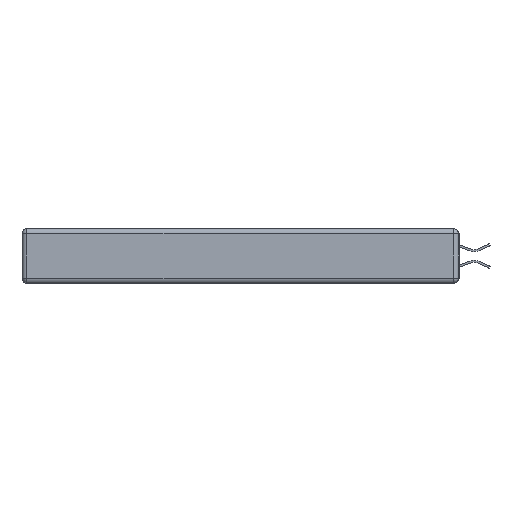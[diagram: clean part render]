
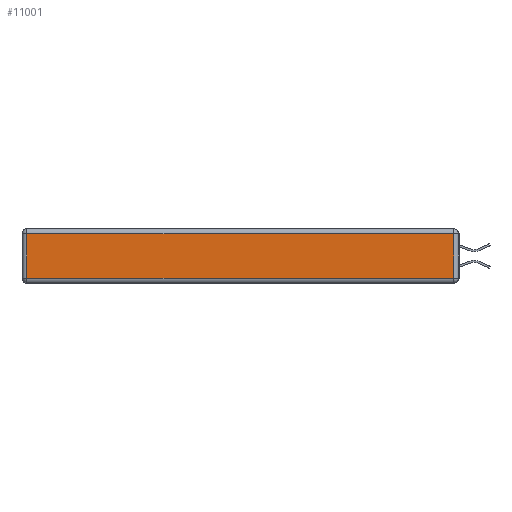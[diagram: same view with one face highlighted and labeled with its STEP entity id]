
A CAD part, left-side view. The second image highlights one B-rep face of the part: STEP entity #11001.
In plain terms, the highlighted planar face has unit normal (-1, 0, 0).
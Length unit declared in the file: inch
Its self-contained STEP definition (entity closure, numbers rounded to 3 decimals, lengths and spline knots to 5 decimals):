
#129 = LINE ( 'NONE', #2565, #17460 ) ;
#185 = FACE_OUTER_BOUND ( 'NONE', #7749, .T. ) ;
#680 = ORIENTED_EDGE ( 'NONE', *, *, #11595, .T. ) ;
#705 = VECTOR ( 'NONE', #15990, 39.37008 ) ;
#1683 = DIRECTION ( 'NONE',  ( 0., 0., -1. ) ) ;
#2207 = VECTOR ( 'NONE', #8833, 39.37008 ) ;
#2259 = CARTESIAN_POINT ( 'NONE',  ( 0., 0.03, -0.03 ) ) ;
#2486 = CARTESIAN_POINT ( 'NONE',  ( 0., 0.03, -0.343 ) ) ;
#2565 = CARTESIAN_POINT ( 'NONE',  ( 0., 2.72, -0.343 ) ) ;
#2656 = DIRECTION ( 'NONE',  ( -1., 0., 0. ) ) ;
#5015 = CARTESIAN_POINT ( 'NONE',  ( 0., 2.72, -0.03 ) ) ;
#5142 = ORIENTED_EDGE ( 'NONE', *, *, #6694, .T. ) ;
#6274 = EDGE_CURVE ( 'NONE', #8579, #17304, #129, .T. ) ;
#6694 = EDGE_CURVE ( 'NONE', #13769, #8579, #16343, .T. ) ;
#7749 = EDGE_LOOP ( 'NONE', ( #680, #15791, #5142, #9722 ) ) ;
#8579 = VERTEX_POINT ( 'NONE', #5015 ) ;
#8601 = LINE ( 'NONE', #2486, #705 ) ;
#8833 = DIRECTION ( 'NONE',  ( 0., 1., 0. ) ) ;
#9507 = AXIS2_PLACEMENT_3D ( 'NONE', #16330, #2656, #13450 ) ;
#9722 = ORIENTED_EDGE ( 'NONE', *, *, #6274, .T. ) ;
#9966 = VECTOR ( 'NONE', #14427, 39.37008 ) ;
#10369 = CARTESIAN_POINT ( 'NONE',  ( 0., 2.75, -0.03 ) ) ;
#11001 = ADVANCED_FACE ( 'NONE', ( #185 ), #17706, .T. ) ;
#11276 = VERTEX_POINT ( 'NONE', #16136 ) ;
#11595 = EDGE_CURVE ( 'NONE', #17304, #11276, #17279, .T. ) ;
#11831 = CARTESIAN_POINT ( 'NONE',  ( 0., 0., -0.313 ) ) ;
#13450 = DIRECTION ( 'NONE',  ( 0., 0., 1. ) ) ;
#13769 = VERTEX_POINT ( 'NONE', #2259 ) ;
#14018 = EDGE_CURVE ( 'NONE', #11276, #13769, #8601, .T. ) ;
#14427 = DIRECTION ( 'NONE',  ( 0., -1., 0. ) ) ;
#15791 = ORIENTED_EDGE ( 'NONE', *, *, #14018, .T. ) ;
#15990 = DIRECTION ( 'NONE',  ( 0., 0., 1. ) ) ;
#16136 = CARTESIAN_POINT ( 'NONE',  ( 0., 0.03, -0.313 ) ) ;
#16330 = CARTESIAN_POINT ( 'NONE',  ( 0., 0., -0.343 ) ) ;
#16343 = LINE ( 'NONE', #10369, #2207 ) ;
#17279 = LINE ( 'NONE', #11831, #9966 ) ;
#17304 = VERTEX_POINT ( 'NONE', #17308 ) ;
#17308 = CARTESIAN_POINT ( 'NONE',  ( 0., 2.72, -0.313 ) ) ;
#17460 = VECTOR ( 'NONE', #1683, 39.37008 ) ;
#17706 = PLANE ( 'NONE',  #9507 ) ;
